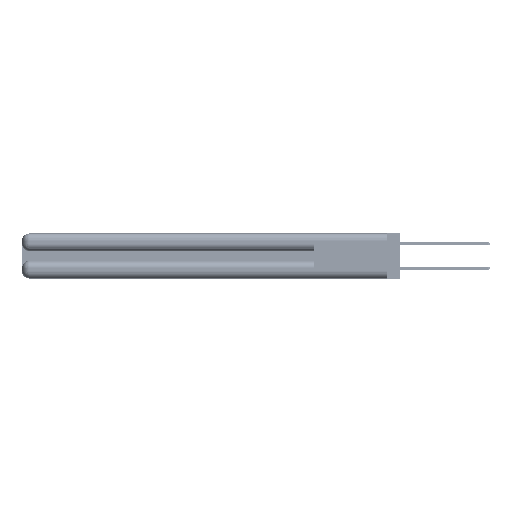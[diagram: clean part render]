
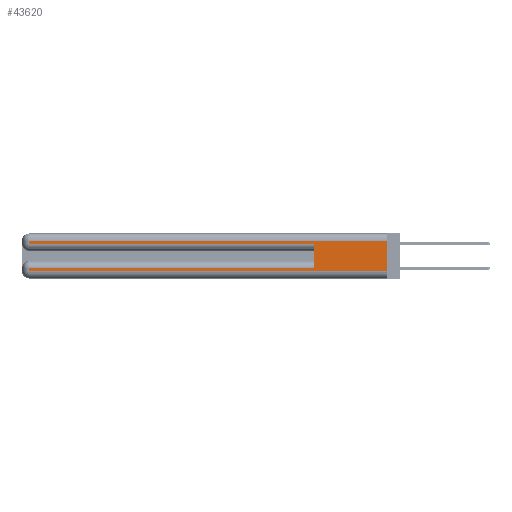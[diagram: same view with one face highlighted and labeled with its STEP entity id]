
A CAD part, left-side view. The second image highlights one B-rep face of the part: STEP entity #43620.
In plain terms, the highlighted planar face has unit normal (-1, 0, 0).
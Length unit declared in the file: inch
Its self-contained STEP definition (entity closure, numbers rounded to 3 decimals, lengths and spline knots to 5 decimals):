
#255 = DIRECTION ( 'NONE',  ( 0., -1., 0. ) ) ;
#902 = FACE_OUTER_BOUND ( 'NONE', #45968, .T. ) ;
#1322 = LINE ( 'NONE', #9134, #35156 ) ;
#1528 = ORIENTED_EDGE ( 'NONE', *, *, #1724, .T. ) ;
#1724 = EDGE_CURVE ( 'NONE', #41914, #27784, #1322, .T. ) ;
#1973 = VECTOR ( 'NONE', #35774, 39.37008 ) ;
#2467 = EDGE_CURVE ( 'NONE', #50317, #3857, #42606, .T. ) ;
#2514 = VECTOR ( 'NONE', #14643, 39.37008 ) ;
#3255 = CARTESIAN_POINT ( 'NONE',  ( 0., 0., 0.06 ) ) ;
#3857 = VERTEX_POINT ( 'NONE', #29344 ) ;
#4004 = CARTESIAN_POINT ( 'NONE',  ( 0., 0.6, 0.285 ) ) ;
#4472 = VERTEX_POINT ( 'NONE', #20996 ) ;
#6307 = ORIENTED_EDGE ( 'NONE', *, *, #29040, .F. ) ;
#7392 = VECTOR ( 'NONE', #39621, 39.37008 ) ;
#9134 = CARTESIAN_POINT ( 'NONE',  ( 0., 0., 0.06 ) ) ;
#11569 = CARTESIAN_POINT ( 'NONE',  ( 0., 0., 0.37 ) ) ;
#11782 = VERTEX_POINT ( 'NONE', #33871 ) ;
#13284 = CARTESIAN_POINT ( 'NONE',  ( 0., 0., 0.37 ) ) ;
#13646 = EDGE_CURVE ( 'NONE', #4472, #39765, #50899, .T. ) ;
#14643 = DIRECTION ( 'NONE',  ( 0., 1., 0. ) ) ;
#15848 = ORIENTED_EDGE ( 'NONE', *, *, #2467, .T. ) ;
#16018 = DIRECTION ( 'NONE',  ( 0., 0., -1. ) ) ;
#18979 = CARTESIAN_POINT ( 'NONE',  ( 0., 2.94, 0.37 ) ) ;
#20546 = VECTOR ( 'NONE', #49843, 39.37008 ) ;
#20996 = CARTESIAN_POINT ( 'NONE',  ( 0., 0.6, 0.085 ) ) ;
#21712 = VERTEX_POINT ( 'NONE', #4004 ) ;
#23344 = CARTESIAN_POINT ( 'NONE',  ( 0., 0., 0.085 ) ) ;
#23501 = ORIENTED_EDGE ( 'NONE', *, *, #42405, .T. ) ;
#23927 = VECTOR ( 'NONE', #44207, 39.37008 ) ;
#24719 = ORIENTED_EDGE ( 'NONE', *, *, #28600, .T. ) ;
#24723 = PLANE ( 'NONE',  #28531 ) ;
#26343 = CARTESIAN_POINT ( 'NONE',  ( 0., 2.94, 0.085 ) ) ;
#26404 = ORIENTED_EDGE ( 'NONE', *, *, #13646, .T. ) ;
#26725 = CARTESIAN_POINT ( 'NONE',  ( 0., 2.94, 0.31 ) ) ;
#27784 = VERTEX_POINT ( 'NONE', #3255 ) ;
#28531 = AXIS2_PLACEMENT_3D ( 'NONE', #11569, #42474, #16018 ) ;
#28600 = EDGE_CURVE ( 'NONE', #11782, #50317, #42698, .T. ) ;
#29040 = EDGE_CURVE ( 'NONE', #4472, #21712, #55747, .T. ) ;
#29344 = CARTESIAN_POINT ( 'NONE',  ( 0., 2.94, 0.285 ) ) ;
#31348 = CARTESIAN_POINT ( 'NONE',  ( 0., 0., 0.285 ) ) ;
#32248 = ORIENTED_EDGE ( 'NONE', *, *, #50928, .F. ) ;
#33755 = ORIENTED_EDGE ( 'NONE', *, *, #46284, .T. ) ;
#33871 = CARTESIAN_POINT ( 'NONE',  ( 0., 0., 0.31 ) ) ;
#34247 = LINE ( 'NONE', #13284, #23927 ) ;
#35113 = DIRECTION ( 'NONE',  ( 0., 0., -1. ) ) ;
#35156 = VECTOR ( 'NONE', #255, 39.37008 ) ;
#35774 = DIRECTION ( 'NONE',  ( 0., -1., 0. ) ) ;
#36193 = CARTESIAN_POINT ( 'NONE',  ( 0., 0., 0.31 ) ) ;
#37195 = LINE ( 'NONE', #31348, #1973 ) ;
#39621 = DIRECTION ( 'NONE',  ( 0., 0., 1. ) ) ;
#39765 = VERTEX_POINT ( 'NONE', #26343 ) ;
#41313 = VECTOR ( 'NONE', #49536, 39.37008 ) ;
#41914 = VERTEX_POINT ( 'NONE', #49285 ) ;
#42405 = EDGE_CURVE ( 'NONE', #39765, #41914, #56265, .T. ) ;
#42474 = DIRECTION ( 'NONE',  ( 1., 0., 0. ) ) ;
#42606 = LINE ( 'NONE', #18979, #20546 ) ;
#42698 = LINE ( 'NONE', #36193, #41313 ) ;
#43620 = ADVANCED_FACE ( 'NONE', ( #902 ), #24723, .F. ) ;
#44207 = DIRECTION ( 'NONE',  ( 0., 0., -1. ) ) ;
#45952 = VECTOR ( 'NONE', #35113, 39.37008 ) ;
#45968 = EDGE_LOOP ( 'NONE', ( #32248, #24719, #15848, #33755, #6307, #26404, #23501, #1528 ) ) ;
#46284 = EDGE_CURVE ( 'NONE', #3857, #21712, #37195, .T. ) ;
#49285 = CARTESIAN_POINT ( 'NONE',  ( 0., 2.94, 0.06 ) ) ;
#49536 = DIRECTION ( 'NONE',  ( 0., 1., 0. ) ) ;
#49843 = DIRECTION ( 'NONE',  ( 0., 0., -1. ) ) ;
#50317 = VERTEX_POINT ( 'NONE', #26725 ) ;
#50899 = LINE ( 'NONE', #23344, #2514 ) ;
#50928 = EDGE_CURVE ( 'NONE', #11782, #27784, #34247, .T. ) ;
#52560 = CARTESIAN_POINT ( 'NONE',  ( 0., 0.6, 0.145 ) ) ;
#55747 = LINE ( 'NONE', #52560, #7392 ) ;
#56265 = LINE ( 'NONE', #57092, #45952 ) ;
#57092 = CARTESIAN_POINT ( 'NONE',  ( 0., 2.94, 0.37 ) ) ;
